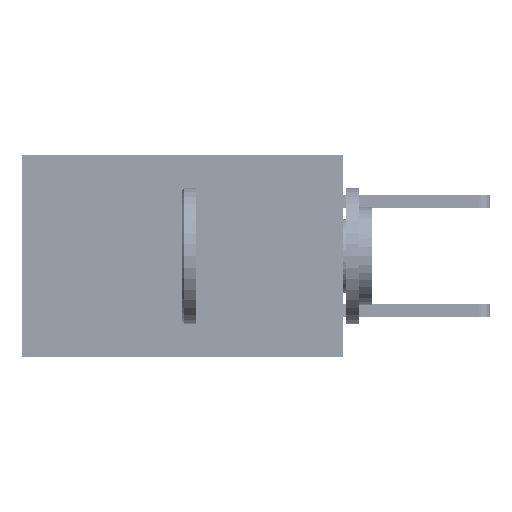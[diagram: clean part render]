
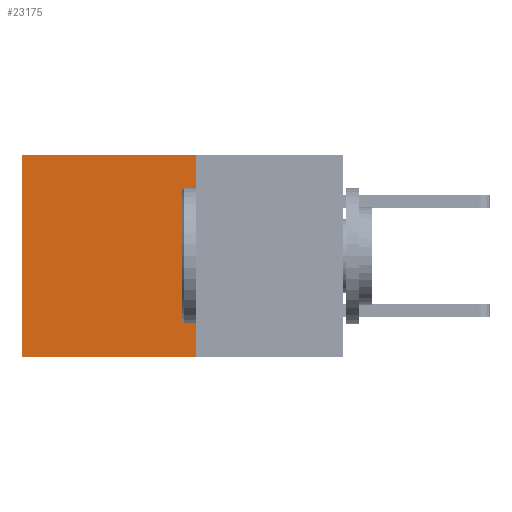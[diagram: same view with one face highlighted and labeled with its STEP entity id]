
A CAD part, left-side view. The second image highlights one B-rep face of the part: STEP entity #23175.
In plain terms, the highlighted planar face has unit normal (-1, 0, 0).
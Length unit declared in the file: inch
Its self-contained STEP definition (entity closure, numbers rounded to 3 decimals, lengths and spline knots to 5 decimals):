
#1 = EDGE_CURVE ( 'NONE', #26616, #7828, #10369, .T. ) ;
#126 = DIRECTION ( 'NONE',  ( 1., 0., 0. ) ) ;
#427 = CARTESIAN_POINT ( 'NONE',  ( 0.277, 0.59, -0.37 ) ) ;
#1786 = VECTOR ( 'NONE', #31451, 39.37008 ) ;
#2599 = CARTESIAN_POINT ( 'NONE',  ( 0.277, 0.27, -0.37 ) ) ;
#2654 = VERTEX_POINT ( 'NONE', #15917 ) ;
#2783 = DIRECTION ( 'NONE',  ( 0., 1., 0. ) ) ;
#3372 = VECTOR ( 'NONE', #19724, 39.37008 ) ;
#4776 = CARTESIAN_POINT ( 'NONE',  ( 0.277, 0.27, 0. ) ) ;
#5286 = FACE_OUTER_BOUND ( 'NONE', #20363, .T. ) ;
#7828 = VERTEX_POINT ( 'NONE', #14668 ) ;
#7974 = LINE ( 'NONE', #12980, #1786 ) ;
#9023 = ORIENTED_EDGE ( 'NONE', *, *, #31844, .T. ) ;
#10369 = LINE ( 'NONE', #2599, #3372 ) ;
#11691 = ORIENTED_EDGE ( 'NONE', *, *, #1, .F. ) ;
#12980 = CARTESIAN_POINT ( 'NONE',  ( 0.277, 0.27, 0. ) ) ;
#13813 = VECTOR ( 'NONE', #2783, 39.37008 ) ;
#14668 = CARTESIAN_POINT ( 'NONE',  ( 0.277, 0.27, -0.37 ) ) ;
#15909 = CARTESIAN_POINT ( 'NONE',  ( 0.277, 0.27, -0.37 ) ) ;
#15917 = CARTESIAN_POINT ( 'NONE',  ( 0.277, 0.59, -0.37 ) ) ;
#15944 = CARTESIAN_POINT ( 'NONE',  ( 0.277, 0.27, -0.37 ) ) ;
#18583 = DIRECTION ( 'NONE',  ( 0., 0., -1. ) ) ;
#19510 = VERTEX_POINT ( 'NONE', #31289 ) ;
#19724 = DIRECTION ( 'NONE',  ( 0., 0., -1. ) ) ;
#20363 = EDGE_LOOP ( 'NONE', ( #9023, #22428, #11691, #31945 ) ) ;
#20796 = EDGE_CURVE ( 'NONE', #7828, #2654, #27849, .T. ) ;
#21426 = EDGE_CURVE ( 'NONE', #26616, #19510, #7974, .T. ) ;
#21542 = DIRECTION ( 'NONE',  ( 0., 0., -1. ) ) ;
#22428 = ORIENTED_EDGE ( 'NONE', *, *, #20796, .F. ) ;
#23175 = ADVANCED_FACE ( 'NONE', ( #5286 ), #29106, .F. ) ;
#26616 = VERTEX_POINT ( 'NONE', #4776 ) ;
#27799 = VECTOR ( 'NONE', #21542, 39.37008 ) ;
#27849 = LINE ( 'NONE', #15909, #13813 ) ;
#28640 = LINE ( 'NONE', #427, #27799 ) ;
#29106 = PLANE ( 'NONE',  #33121 ) ;
#31289 = CARTESIAN_POINT ( 'NONE',  ( 0.277, 0.59, 0. ) ) ;
#31451 = DIRECTION ( 'NONE',  ( 0., 1., 0. ) ) ;
#31844 = EDGE_CURVE ( 'NONE', #19510, #2654, #28640, .T. ) ;
#31945 = ORIENTED_EDGE ( 'NONE', *, *, #21426, .T. ) ;
#33121 = AXIS2_PLACEMENT_3D ( 'NONE', #15944, #126, #18583 ) ;
